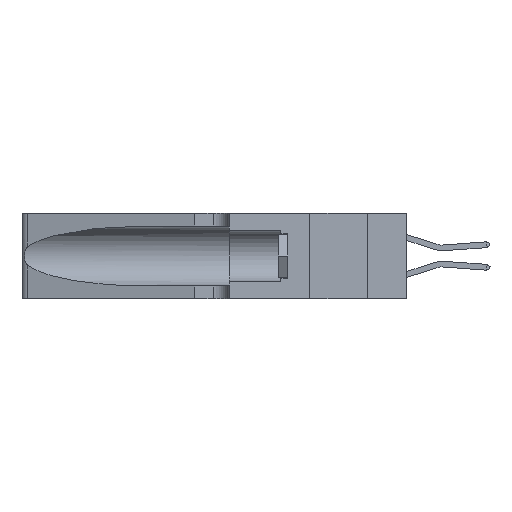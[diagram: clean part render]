
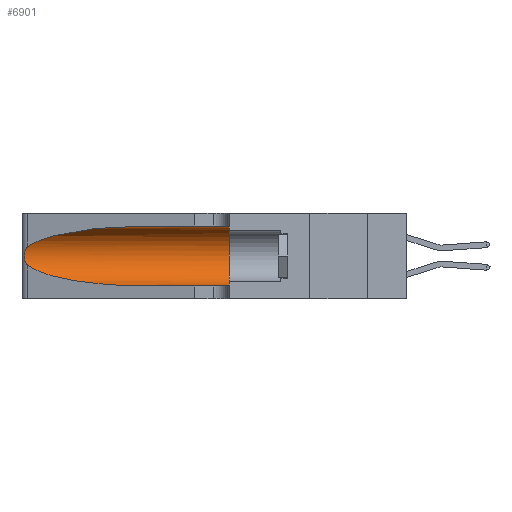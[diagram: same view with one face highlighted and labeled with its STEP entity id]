
A CAD part, left-side view. The second image highlights one B-rep face of the part: STEP entity #6901.
In plain terms, the highlighted cylindrical face has radius 3.308 mm (diameter 6.617 mm), a partial arc.
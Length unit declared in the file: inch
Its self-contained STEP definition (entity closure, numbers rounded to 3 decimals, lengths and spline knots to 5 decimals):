
#385 = CARTESIAN_POINT ( 'NONE',  ( 0.25639, 1.23184, 0.21858 ) ) ;
#626 = CARTESIAN_POINT ( 'NONE',  ( 0.25487, 1.22718, 0.14631 ) ) ;
#889 = FACE_OUTER_BOUND ( 'NONE', #15306, .T. ) ;
#1803 = ORIENTED_EDGE ( 'NONE', *, *, #8061, .F. ) ;
#1876 = EDGE_CURVE ( 'NONE', #19539, #14026, #15251, .T. ) ;
#2290 = CARTESIAN_POINT ( 'NONE',  ( 0.1305, 1.61858, 0.185 ) ) ;
#2972 = EDGE_CURVE ( 'NONE', #21460, #24545, #9331, .T. ) ;
#3344 = CARTESIAN_POINT ( 'NONE',  ( 0.25856, 1.23593, 0.16098 ) ) ;
#3369 = CARTESIAN_POINT ( 'NONE',  ( 0.18966, 0.96281, 0.05475 ) ) ;
#4007 = CARTESIAN_POINT ( 'NONE',  ( 0.1305, 0.72297, 0.31525 ) ) ;
#4331 = CARTESIAN_POINT ( 'NONE',  ( 0.1305, 1.61858, 0.31525 ) ) ;
#4455 = DIRECTION ( 'NONE',  ( 0., -1., 0. ) ) ;
#5027 = ORIENTED_EDGE ( 'NONE', *, *, #32901, .T. ) ;
#5525 = CYLINDRICAL_SURFACE ( 'NONE', #25342, 0.13025 ) ;
#5714 = CARTESIAN_POINT ( 'NONE',  ( 0.25487, 1.22718, 0.22369 ) ) ;
#5824 = CARTESIAN_POINT ( 'NONE',  ( 0.25787, 1.23484, 0.2124 ) ) ;
#6259 = CARTESIAN_POINT ( 'NONE',  ( 0.1305, 0.72297, 0.05475 ) ) ;
#6382 = CARTESIAN_POINT ( 'NONE',  ( 0.1305, 0.35, 0.05475 ) ) ;
#6404 = CARTESIAN_POINT ( 'NONE',  ( 0.25555, 1.22993, 0.14849 ) ) ;
#6901 = ADVANCED_FACE ( 'NONE', ( #889 ), #5525, .F. ) ;
#6997 = ORIENTED_EDGE ( 'NONE', *, *, #2972, .T. ) ;
#8061 = EDGE_CURVE ( 'NONE', #17505, #27450, #28885, .T. ) ;
#8403 = CARTESIAN_POINT ( 'NONE',  ( 0.25555, 1.22994, 0.2215 ) ) ;
#8997 = CARTESIAN_POINT ( 'NONE',  ( 0.26018, 1.23835, 0.19895 ) ) ;
#9223 = CARTESIAN_POINT ( 'NONE',  ( 0.25639, 1.23186, 0.15144 ) ) ;
#9331 = LINE ( 'NONE', #32365, #28169 ) ;
#9503 = CARTESIAN_POINT ( 'NONE',  ( 0.18966, 0.96281, 0.31525 ) ) ;
#10014 = EDGE_CURVE ( 'NONE', #27450, #24545, #20870, .T. ) ;
#10105 = DIRECTION ( 'NONE',  ( 0., 0., 1. ) ) ;
#10241 = CARTESIAN_POINT ( 'NONE',  ( 0.1305, 0.35, 0.31525 ) ) ;
#11365 = CARTESIAN_POINT ( 'NONE',  ( 0.25487, 1.22718, 0.14631 ) ) ;
#11374 = ORIENTED_EDGE ( 'NONE', *, *, #19989, .T. ) ;
#11904 = CARTESIAN_POINT ( 'NONE',  ( 0.26075, 1.23896, 0.19203 ) ) ;
#12319 = CARTESIAN_POINT ( 'NONE',  ( 0.25487, 1.22718, 0.22369 ) ) ;
#13210 = DIRECTION ( 'NONE',  ( 0., -1., 0. ) ) ;
#14026 = VERTEX_POINT ( 'NONE', #25851 ) ;
#14952 = CARTESIAN_POINT ( 'NONE',  ( 0.1305, 0.72297, 0.31525 ) ) ;
#15251 = B_SPLINE_CURVE_WITH_KNOTS ( 'NONE', 3,
 ( #5714, #8403, #385, #5824, #22347, #8997, #11904, #22464, #33312, #3344, #17152, #9223, #6404, #626 ),
 .UNSPECIFIED., .F., .F.,
 ( 4, 2, 2, 2, 2, 2, 4 ),
 ( 0., 0.00027, 0.00053, 0.00107, 0.0016, 0.00187, 0.00214 ),
 .UNSPECIFIED. ) ;
#15306 = EDGE_LOOP ( 'NONE', ( #5027, #34374, #11374, #6997, #24449, #1803 ) ) ;
#17152 = CARTESIAN_POINT ( 'NONE',  ( 0.25789, 1.23486, 0.15765 ) ) ;
#17505 = VERTEX_POINT ( 'NONE', #4007 ) ;
#19539 = VERTEX_POINT ( 'NONE', #12319 ) ;
#19989 = EDGE_CURVE ( 'NONE', #14026, #21460, #30650, .T. ) ;
#20870 = CIRCLE ( 'NONE', #27644, 0.13025 ) ;
#20968 = CARTESIAN_POINT ( 'NONE',  ( 0.1305, 0.35, 0.185 ) ) ;
#21460 = VERTEX_POINT ( 'NONE', #6259 ) ;
#21790 = VECTOR ( 'NONE', #4455, 39.37008 ) ;
#22347 = CARTESIAN_POINT ( 'NONE',  ( 0.25854, 1.2359, 0.20912 ) ) ;
#22464 = CARTESIAN_POINT ( 'NONE',  ( 0.26075, 1.23896, 0.178 ) ) ;
#23002 =( BOUNDED_CURVE ( )  B_SPLINE_CURVE ( 3, ( #14952, #9503, #28203, #25283 ),
 .UNSPECIFIED., .F., .F. ) 
 B_SPLINE_CURVE_WITH_KNOTS ( ( 4, 4 ),
 ( 1.5708, 2.84003 ),
 .UNSPECIFIED. ) 
 CURVE ( )  GEOMETRIC_REPRESENTATION_ITEM ( )  RATIONAL_B_SPLINE_CURVE ( ( 1., 0.87, 0.87, 1. ) ) 
 REPRESENTATION_ITEM ( '' )  );
#24449 = ORIENTED_EDGE ( 'NONE', *, *, #10014, .F. ) ;
#24545 = VERTEX_POINT ( 'NONE', #6382 ) ;
#24709 = CARTESIAN_POINT ( 'NONE',  ( 0.2373, 1.15595, 0.08982 ) ) ;
#24944 = CARTESIAN_POINT ( 'NONE',  ( 0.1305, 0.72297, 0.05475 ) ) ;
#25283 = CARTESIAN_POINT ( 'NONE',  ( 0.25487, 1.22718, 0.22369 ) ) ;
#25342 = AXIS2_PLACEMENT_3D ( 'NONE', #2290, #13210, #34500 ) ;
#25851 = CARTESIAN_POINT ( 'NONE',  ( 0.25487, 1.22718, 0.14631 ) ) ;
#25997 = DIRECTION ( 'NONE',  ( 0., 1., 0. ) ) ;
#26620 = DIRECTION ( 'NONE',  ( 0., -1., 0. ) ) ;
#27450 = VERTEX_POINT ( 'NONE', #10241 ) ;
#27644 = AXIS2_PLACEMENT_3D ( 'NONE', #20968, #25997, #10105 ) ;
#28169 = VECTOR ( 'NONE', #26620, 39.37008 ) ;
#28203 = CARTESIAN_POINT ( 'NONE',  ( 0.2373, 1.15595, 0.28018 ) ) ;
#28885 = LINE ( 'NONE', #4331, #21790 ) ;
#30650 =( BOUNDED_CURVE ( )  B_SPLINE_CURVE ( 3, ( #11365, #24709, #3369, #24944 ),
 .UNSPECIFIED., .F., .F. ) 
 B_SPLINE_CURVE_WITH_KNOTS ( ( 4, 4 ),
 ( 3.44316, 4.71239 ),
 .UNSPECIFIED. ) 
 CURVE ( )  GEOMETRIC_REPRESENTATION_ITEM ( )  RATIONAL_B_SPLINE_CURVE ( ( 1., 0.87, 0.87, 1. ) ) 
 REPRESENTATION_ITEM ( '' )  );
#32365 = CARTESIAN_POINT ( 'NONE',  ( 0.1305, 1.61858, 0.05475 ) ) ;
#32901 = EDGE_CURVE ( 'NONE', #17505, #19539, #23002, .T. ) ;
#33312 = CARTESIAN_POINT ( 'NONE',  ( 0.26017, 1.23833, 0.17102 ) ) ;
#34374 = ORIENTED_EDGE ( 'NONE', *, *, #1876, .T. ) ;
#34500 = DIRECTION ( 'NONE',  ( 0., 0., -1. ) ) ;
